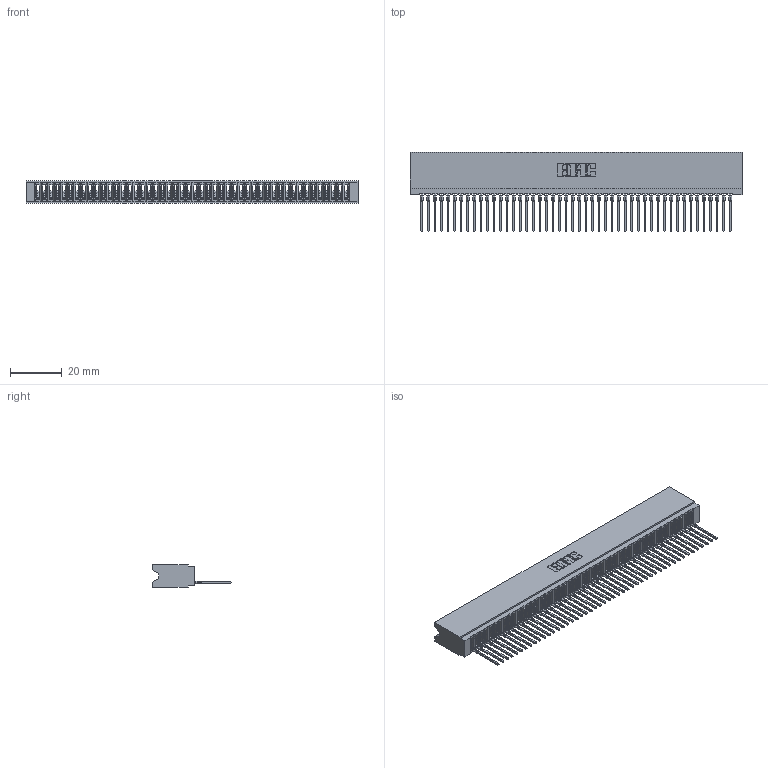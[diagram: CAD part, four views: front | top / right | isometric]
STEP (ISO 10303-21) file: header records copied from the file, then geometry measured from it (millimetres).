
FILE_DESCRIPTION (( 'STEP AP203' ), '1' );
FILE_NAME ('745-048-545-106.STEP', '2026-02-25T21:36:29', ( '' ), ( '' ), 'SwSTEP 2.0', 'SolidWorks 2023', '' );
FILE_SCHEMA (( 'CONFIG_CONTROL_DESIGN' ));
Length unit declared in the file: millimetre
Products named in the file (3): 745 Part_Insulator Option - 06; 745-292-001_545; 745-048-545-106
Assembly tree (49 placements, depth 2):
  745-048-545-106
    745 Part_Insulator Option - 06
    745-292-001_545  x48
Bounding box: 128.52 x 30.62 x 8.89 mm (x, y, z)
Volume: 11214.2 mm3; surface area: 21746.4 mm2
Topology: 49 solids, 49 shells, 5472 faces, 15044 edges, 9484 vertices
Faces by surface type: plane 3272, bspline 960, cylinder 952, torus 288
Entity records: 78474 total; most frequent: CARTESIAN_POINT 14330, ORIENTED_EDGE 13826, DIRECTION 11977, EDGE_CURVE 6913, VECTOR 6443, LINE 6443, VERTEX_POINT 4408, AXIS2_PLACEMENT_3D 2767
